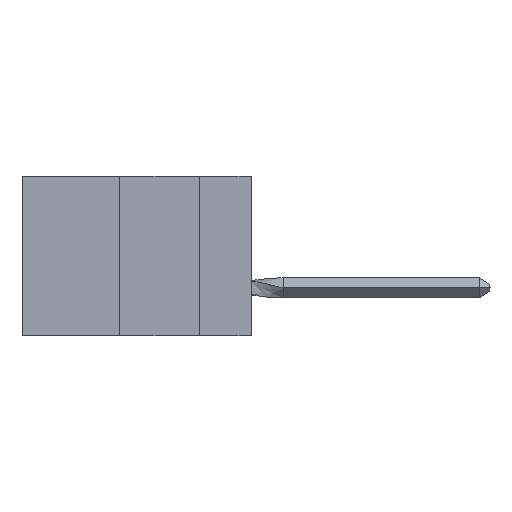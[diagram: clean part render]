
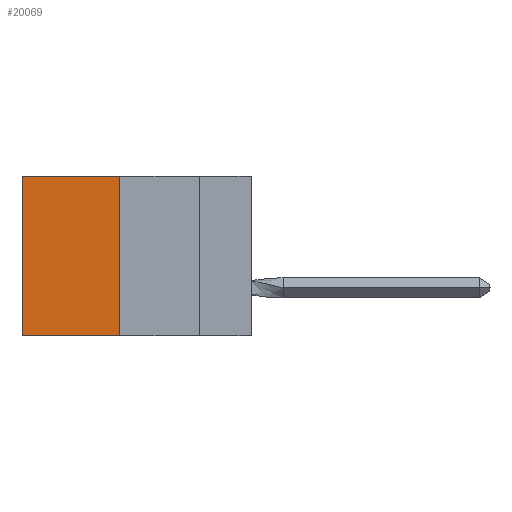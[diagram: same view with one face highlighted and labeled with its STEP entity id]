
A CAD part, left-side view. The second image highlights one B-rep face of the part: STEP entity #20069.
In plain terms, the highlighted planar face has unit normal (-1, 0, 0).
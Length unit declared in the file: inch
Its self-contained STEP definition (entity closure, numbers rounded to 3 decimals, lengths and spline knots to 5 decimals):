
#336 = DIRECTION ( 'NONE',  ( 0., 0., -1. ) ) ;
#563 = VECTOR ( 'NONE', #336, 39.37008 ) ;
#767 = PLANE ( 'NONE',  #27440 ) ;
#1230 = VECTOR ( 'NONE', #25320, 39.37008 ) ;
#2365 = LINE ( 'NONE', #9902, #563 ) ;
#2431 = VERTEX_POINT ( 'NONE', #6287 ) ;
#4407 = EDGE_CURVE ( 'NONE', #26032, #2431, #2365, .T. ) ;
#5056 = DIRECTION ( 'NONE',  ( 0., 1., 0. ) ) ;
#6056 = CARTESIAN_POINT ( 'NONE',  ( 0.305, 0.413, -0.5 ) ) ;
#6287 = CARTESIAN_POINT ( 'NONE',  ( 0.305, 0.72, -0.5 ) ) ;
#6487 = VECTOR ( 'NONE', #13158, 39.37008 ) ;
#9902 = CARTESIAN_POINT ( 'NONE',  ( 0.305, 0.72, -0.5 ) ) ;
#11333 = ORIENTED_EDGE ( 'NONE', *, *, #18885, .F. ) ;
#11512 = LINE ( 'NONE', #24141, #27937 ) ;
#11575 = FACE_OUTER_BOUND ( 'NONE', #27531, .T. ) ;
#12320 = EDGE_CURVE ( 'NONE', #17474, #21989, #14193, .T. ) ;
#13158 = DIRECTION ( 'NONE',  ( 0., 0., -1. ) ) ;
#13701 = CARTESIAN_POINT ( 'NONE',  ( 0.305, 0.413, 0. ) ) ;
#13819 = CARTESIAN_POINT ( 'NONE',  ( 0.305, 0.72, 0. ) ) ;
#14193 = LINE ( 'NONE', #17737, #6487 ) ;
#15059 = DIRECTION ( 'NONE',  ( 0., 0., -1. ) ) ;
#15369 = ORIENTED_EDGE ( 'NONE', *, *, #12320, .F. ) ;
#16706 = ORIENTED_EDGE ( 'NONE', *, *, #29796, .T. ) ;
#17474 = VERTEX_POINT ( 'NONE', #26040 ) ;
#17597 = ORIENTED_EDGE ( 'NONE', *, *, #4407, .T. ) ;
#17685 = DIRECTION ( 'NONE',  ( 1., 0., 0. ) ) ;
#17737 = CARTESIAN_POINT ( 'NONE',  ( 0.305, 0.413, -0.5 ) ) ;
#18885 = EDGE_CURVE ( 'NONE', #21989, #2431, #11512, .T. ) ;
#20069 = ADVANCED_FACE ( 'NONE', ( #11575 ), #767, .F. ) ;
#21989 = VERTEX_POINT ( 'NONE', #24209 ) ;
#24141 = CARTESIAN_POINT ( 'NONE',  ( 0.305, 0.413, -0.5 ) ) ;
#24209 = CARTESIAN_POINT ( 'NONE',  ( 0.305, 0.413, -0.5 ) ) ;
#24257 = LINE ( 'NONE', #13701, #1230 ) ;
#25320 = DIRECTION ( 'NONE',  ( 0., 1., 0. ) ) ;
#26032 = VERTEX_POINT ( 'NONE', #13819 ) ;
#26040 = CARTESIAN_POINT ( 'NONE',  ( 0.305, 0.413, 0. ) ) ;
#27440 = AXIS2_PLACEMENT_3D ( 'NONE', #6056, #17685, #15059 ) ;
#27531 = EDGE_LOOP ( 'NONE', ( #17597, #11333, #15369, #16706 ) ) ;
#27937 = VECTOR ( 'NONE', #5056, 39.37008 ) ;
#29796 = EDGE_CURVE ( 'NONE', #17474, #26032, #24257, .T. ) ;
